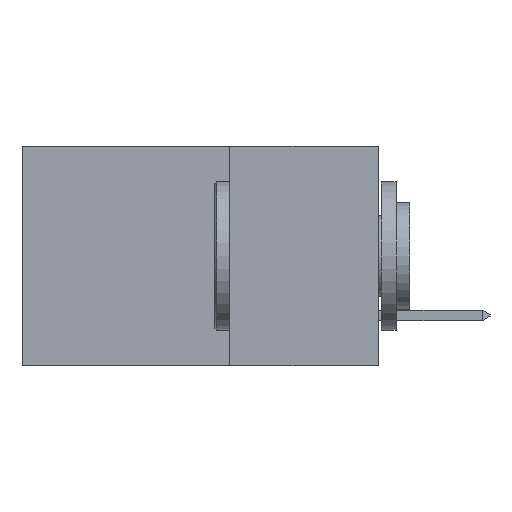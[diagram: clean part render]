
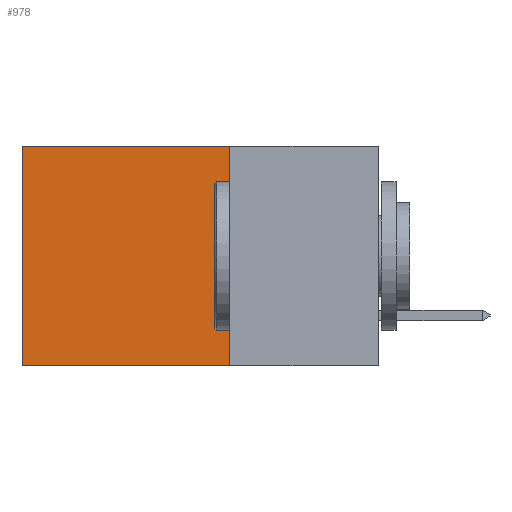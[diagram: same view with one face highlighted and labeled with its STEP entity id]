
A CAD part, left-side view. The second image highlights one B-rep face of the part: STEP entity #978.
In plain terms, the highlighted planar face has unit normal (-1, 0, 0).
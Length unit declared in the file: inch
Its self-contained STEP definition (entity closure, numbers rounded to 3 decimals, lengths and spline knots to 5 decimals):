
#234 = VERTEX_POINT ( 'NONE', #2387 ) ;
#505 = VERTEX_POINT ( 'NONE', #18888 ) ;
#978 = ADVANCED_FACE ( 'NONE', ( #15241 ), #4387, .F. ) ;
#2138 = DIRECTION ( 'NONE',  ( 0., 1., 0. ) ) ;
#2249 = LINE ( 'NONE', #8486, #9413 ) ;
#2387 = CARTESIAN_POINT ( 'NONE',  ( 0.298, 0.25, -0.37 ) ) ;
#3924 = EDGE_CURVE ( 'NONE', #7433, #14640, #5311, .T. ) ;
#4075 = VECTOR ( 'NONE', #10581, 39.37008 ) ;
#4084 = AXIS2_PLACEMENT_3D ( 'NONE', #12707, #10737, #13511 ) ;
#4387 = PLANE ( 'NONE',  #4084 ) ;
#4848 = VECTOR ( 'NONE', #2138, 39.37008 ) ;
#5285 = LINE ( 'NONE', #16279, #9309 ) ;
#5311 = LINE ( 'NONE', #14244, #4848 ) ;
#5335 = ORIENTED_EDGE ( 'NONE', *, *, #3924, .T. ) ;
#7433 = VERTEX_POINT ( 'NONE', #17668 ) ;
#7649 = LINE ( 'NONE', #18162, #4075 ) ;
#8486 = CARTESIAN_POINT ( 'NONE',  ( 0.298, 0.25, 0. ) ) ;
#8657 = EDGE_CURVE ( 'NONE', #7433, #234, #2249, .T. ) ;
#8982 = EDGE_LOOP ( 'NONE', ( #15527, #18006, #11416, #5335 ) ) ;
#9309 = VECTOR ( 'NONE', #13164, 39.37008 ) ;
#9413 = VECTOR ( 'NONE', #17619, 39.37008 ) ;
#9996 = CARTESIAN_POINT ( 'NONE',  ( 0.298, 0.6, 0. ) ) ;
#10581 = DIRECTION ( 'NONE',  ( 0., 0., -1. ) ) ;
#10737 = DIRECTION ( 'NONE',  ( 1., 0., 0. ) ) ;
#11167 = EDGE_CURVE ( 'NONE', #14640, #505, #7649, .T. ) ;
#11416 = ORIENTED_EDGE ( 'NONE', *, *, #8657, .F. ) ;
#12707 = CARTESIAN_POINT ( 'NONE',  ( 0.298, 0.25, 0. ) ) ;
#12856 = EDGE_CURVE ( 'NONE', #234, #505, #5285, .T. ) ;
#13164 = DIRECTION ( 'NONE',  ( 0., 1., 0. ) ) ;
#13511 = DIRECTION ( 'NONE',  ( 0., 0., -1. ) ) ;
#14244 = CARTESIAN_POINT ( 'NONE',  ( 0.298, 0.25, 0. ) ) ;
#14640 = VERTEX_POINT ( 'NONE', #9996 ) ;
#15241 = FACE_OUTER_BOUND ( 'NONE', #8982, .T. ) ;
#15527 = ORIENTED_EDGE ( 'NONE', *, *, #11167, .T. ) ;
#16279 = CARTESIAN_POINT ( 'NONE',  ( 0.298, 0.25, -0.37 ) ) ;
#17619 = DIRECTION ( 'NONE',  ( 0., 0., -1. ) ) ;
#17668 = CARTESIAN_POINT ( 'NONE',  ( 0.298, 0.25, 0. ) ) ;
#18006 = ORIENTED_EDGE ( 'NONE', *, *, #12856, .F. ) ;
#18162 = CARTESIAN_POINT ( 'NONE',  ( 0.298, 0.6, 0. ) ) ;
#18888 = CARTESIAN_POINT ( 'NONE',  ( 0.298, 0.6, -0.37 ) ) ;
